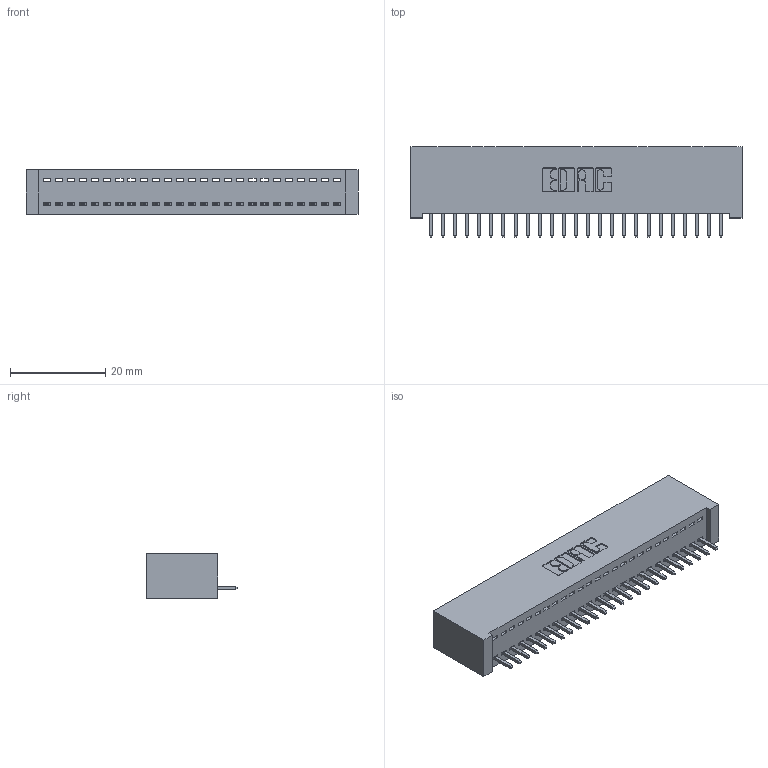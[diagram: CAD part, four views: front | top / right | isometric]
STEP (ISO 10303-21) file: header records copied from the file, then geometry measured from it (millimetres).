
FILE_DESCRIPTION (( 'STEP AP203' ), '1' );
FILE_NAME ('342-025-521-101.STEP', '2018-08-11T03:17:32', ( '' ), ( '' ), 'SwSTEP 2.0', 'SolidWorks 2016', '' );
FILE_SCHEMA (( 'CONFIG_CONTROL_DESIGN' ));
Length unit declared in the file: inch
Products named in the file (3): 342 Part_Lugless; 345-292-001_345-293-121; 342-025-521-101
Assembly tree (26 placements, depth 2):
  342-025-521-101
    342 Part_Lugless
    345-292-001_345-293-121  x25
Bounding box: 69.75 x 19.06 x 9.4 mm (x, y, z)
Volume: 6390.8 mm3; surface area: 9117.4 mm2
Topology: 26 solids, 26 shells, 1552 faces, 4675 edges, 3082 vertices
Faces by surface type: plane 1112, cylinder 440
Entity records: 17091 total; most frequent: CARTESIAN_POINT 2957, ORIENTED_EDGE 2918, DIRECTION 2521, EDGE_CURVE 1459, LINE 1339, VECTOR 1339, VERTEX_POINT 970, AXIS2_PLACEMENT_3D 591
